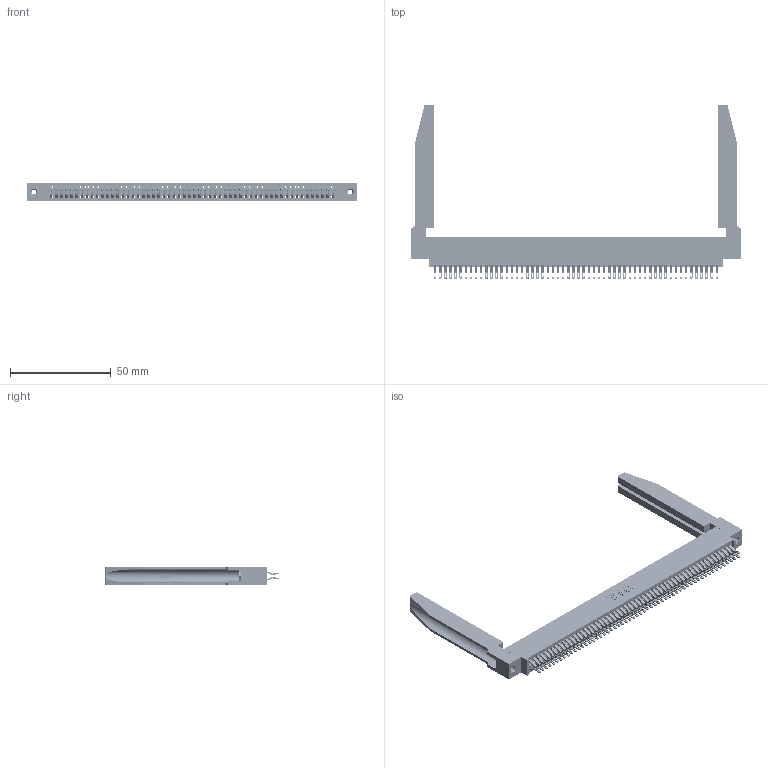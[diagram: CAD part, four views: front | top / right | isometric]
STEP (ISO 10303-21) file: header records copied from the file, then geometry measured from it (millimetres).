
FILE_DESCRIPTION (( 'STEP AP203' ), '1' );
FILE_NAME ('345-112-555-878.STEP', '2019-11-04T22:57:09', ( '' ), ( '' ), 'SwSTEP 2.0', 'SolidWorks 2016', '' );
FILE_SCHEMA (( 'CONFIG_CONTROL_DESIGN' ));
Length unit declared in the file: inch
Products named in the file (5): 345-220-078_345-220-078; 345 Part_0.170 Offset - 0.156 Dia-TH; 345-250-001_345-250-001-102; 345-292-001_555 Tail; 345-112-555-878
Assembly tree (117 placements, depth 2):
  345-112-555-878
    345 Part_0.170 Offset - 0.156 Dia-TH
    345-292-001_555 Tail  x112
    345-250-001_345-250-001-102  x2
    345-220-078_345-220-078  x2
Bounding box: 163.47 x 86.41 x 9.4 mm (x, y, z)
Volume: 23991.9 mm3; surface area: 32361.1 mm2
Topology: 117 solids, 117 shells, 6636 faces, 20785 edges, 13846 vertices
Faces by surface type: plane 3698, cylinder 2886, bspline 36, cone 12, torus 4
Entity records: 47252 total; most frequent: CARTESIAN_POINT 8861, ORIENTED_EDGE 7662, DIRECTION 6757, EDGE_CURVE 3831, LINE 3361, VECTOR 3361, VERTEX_POINT 2548, AXIS2_PLACEMENT_3D 1698
